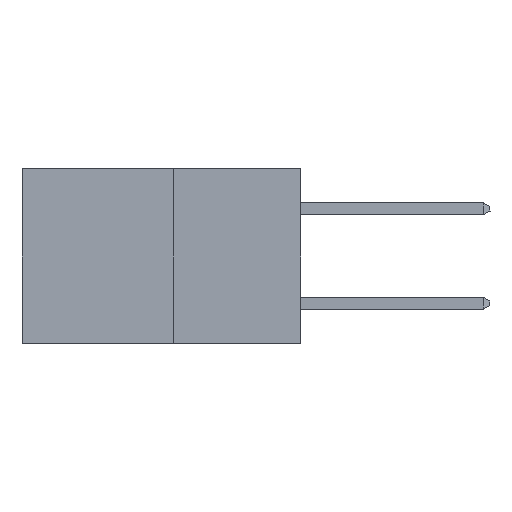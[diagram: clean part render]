
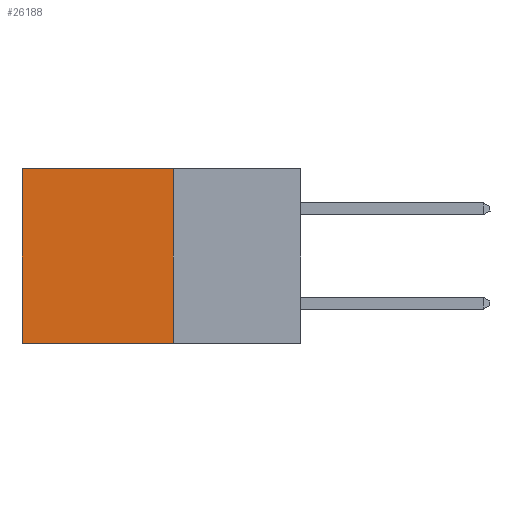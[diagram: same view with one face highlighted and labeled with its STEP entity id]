
A CAD part, left-side view. The second image highlights one B-rep face of the part: STEP entity #26188.
In plain terms, the highlighted planar face has unit normal (-1, 0, 0).
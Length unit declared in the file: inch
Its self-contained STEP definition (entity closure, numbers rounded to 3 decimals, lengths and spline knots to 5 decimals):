
#18 = CARTESIAN_POINT ( 'NONE',  ( 0.277, 0.27, -0.37 ) ) ;
#1133 = LINE ( 'NONE', #15175, #26495 ) ;
#1518 = LINE ( 'NONE', #7452, #5709 ) ;
#2504 = CARTESIAN_POINT ( 'NONE',  ( 0.277, 0.27, -0.37 ) ) ;
#2982 = ORIENTED_EDGE ( 'NONE', *, *, #6651, .T. ) ;
#3408 = DIRECTION ( 'NONE',  ( 0., 0., -1. ) ) ;
#3412 = AXIS2_PLACEMENT_3D ( 'NONE', #18, #8305, #22693 ) ;
#4141 = PLANE ( 'NONE',  #3412 ) ;
#4977 = CARTESIAN_POINT ( 'NONE',  ( 0.277, 0.27, 0. ) ) ;
#5709 = VECTOR ( 'NONE', #3408, 39.37008 ) ;
#6027 = CARTESIAN_POINT ( 'NONE',  ( 0.277, 0.27, -0.37 ) ) ;
#6651 = EDGE_CURVE ( 'NONE', #20150, #11333, #10526, .T. ) ;
#7037 = VECTOR ( 'NONE', #20453, 39.37008 ) ;
#7452 = CARTESIAN_POINT ( 'NONE',  ( 0.277, 0.59, -0.37 ) ) ;
#8305 = DIRECTION ( 'NONE',  ( 1., 0., 0. ) ) ;
#10493 = CARTESIAN_POINT ( 'NONE',  ( 0.277, 0.27, 0. ) ) ;
#10526 = LINE ( 'NONE', #4977, #11207 ) ;
#11132 = DIRECTION ( 'NONE',  ( 0., 1., 0. ) ) ;
#11207 = VECTOR ( 'NONE', #19412, 39.37008 ) ;
#11333 = VERTEX_POINT ( 'NONE', #26300 ) ;
#11714 = VERTEX_POINT ( 'NONE', #21329 ) ;
#12638 = ORIENTED_EDGE ( 'NONE', *, *, #16293, .F. ) ;
#15175 = CARTESIAN_POINT ( 'NONE',  ( 0.277, 0.27, -0.37 ) ) ;
#16293 = EDGE_CURVE ( 'NONE', #20150, #24010, #23472, .T. ) ;
#16571 = ORIENTED_EDGE ( 'NONE', *, *, #18400, .F. ) ;
#16794 = EDGE_CURVE ( 'NONE', #11333, #11714, #1518, .T. ) ;
#18400 = EDGE_CURVE ( 'NONE', #24010, #11714, #1133, .T. ) ;
#19387 = EDGE_LOOP ( 'NONE', ( #23820, #16571, #12638, #2982 ) ) ;
#19412 = DIRECTION ( 'NONE',  ( 0., 1., 0. ) ) ;
#20150 = VERTEX_POINT ( 'NONE', #10493 ) ;
#20453 = DIRECTION ( 'NONE',  ( 0., 0., -1. ) ) ;
#21329 = CARTESIAN_POINT ( 'NONE',  ( 0.277, 0.59, -0.37 ) ) ;
#22693 = DIRECTION ( 'NONE',  ( 0., 0., -1. ) ) ;
#23472 = LINE ( 'NONE', #6027, #7037 ) ;
#23820 = ORIENTED_EDGE ( 'NONE', *, *, #16794, .T. ) ;
#24010 = VERTEX_POINT ( 'NONE', #2504 ) ;
#25143 = FACE_OUTER_BOUND ( 'NONE', #19387, .T. ) ;
#26188 = ADVANCED_FACE ( 'NONE', ( #25143 ), #4141, .F. ) ;
#26300 = CARTESIAN_POINT ( 'NONE',  ( 0.277, 0.59, 0. ) ) ;
#26495 = VECTOR ( 'NONE', #11132, 39.37008 ) ;
